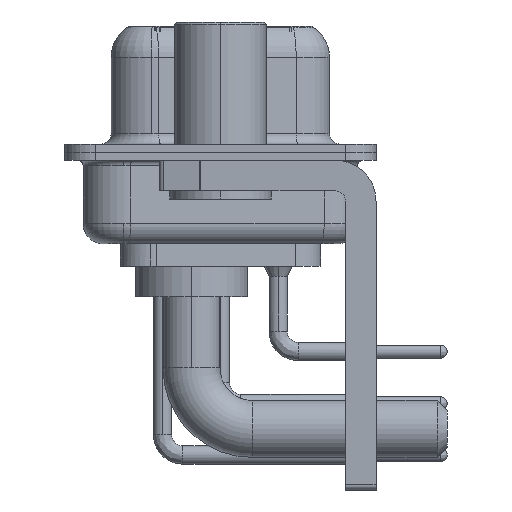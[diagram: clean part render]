
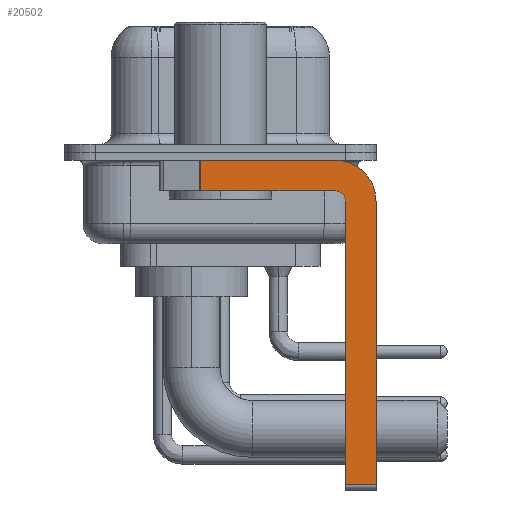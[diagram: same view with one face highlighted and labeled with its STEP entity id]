
A CAD part, left-side view. The second image highlights one B-rep face of the part: STEP entity #20502.
In plain terms, the highlighted planar face has unit normal (-1, 0, 0).
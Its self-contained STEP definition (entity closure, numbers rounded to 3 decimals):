
#913 = DIRECTION ( 'NONE',  ( 0., -1., 0. ) ) ;
#934 = EDGE_CURVE ( 'NONE', #23115, #18921, #5626, .T. ) ;
#1726 = LINE ( 'NONE', #9877, #5058 ) ;
#2110 = VECTOR ( 'NONE', #8054, 1000. ) ;
#2302 = CARTESIAN_POINT ( 'NONE',  ( -2.9, 0.978, -1.9 ) ) ;
#2614 = PLANE ( 'NONE',  #9915 ) ;
#3159 = CARTESIAN_POINT ( 'NONE',  ( -2.9, -7.65, -2.4 ) ) ;
#3480 = CARTESIAN_POINT ( 'NONE',  ( -2.9, -6.15, -16.35 ) ) ;
#3906 = LINE ( 'NONE', #9406, #14219 ) ;
#4399 = DIRECTION ( 'NONE',  ( -1., 0., 0. ) ) ;
#5058 = VECTOR ( 'NONE', #31513, 1000. ) ;
#5063 = ORIENTED_EDGE ( 'NONE', *, *, #16110, .F. ) ;
#5534 = ORIENTED_EDGE ( 'NONE', *, *, #23836, .F. ) ;
#5611 = ORIENTED_EDGE ( 'NONE', *, *, #25659, .F. ) ;
#5626 = LINE ( 'NONE', #13960, #27375 ) ;
#6168 = LINE ( 'NONE', #3159, #31356 ) ;
#7317 = EDGE_CURVE ( 'NONE', #24608, #19240, #34687, .T. ) ;
#7990 = DIRECTION ( 'NONE',  ( 0., 0., -1. ) ) ;
#8054 = DIRECTION ( 'NONE',  ( 0., 0., 1. ) ) ;
#9406 = CARTESIAN_POINT ( 'NONE',  ( -2.9, 3., -0.4 ) ) ;
#9877 = CARTESIAN_POINT ( 'NONE',  ( -2.9, -5.65, -1.9 ) ) ;
#9915 = AXIS2_PLACEMENT_3D ( 'NONE', #18943, #29733, #31865 ) ;
#12101 = ORIENTED_EDGE ( 'NONE', *, *, #7317, .T. ) ;
#12862 = LINE ( 'NONE', #24046, #2110 ) ;
#13932 = ORIENTED_EDGE ( 'NONE', *, *, #934, .T. ) ;
#13960 = CARTESIAN_POINT ( 'NONE',  ( -2.9, 0.978, -1.9 ) ) ;
#14006 = VERTEX_POINT ( 'NONE', #34419 ) ;
#14129 = DIRECTION ( 'NONE',  ( 0., 0., -1. ) ) ;
#14219 = VECTOR ( 'NONE', #913, 1000. ) ;
#14566 = CIRCLE ( 'NONE', #28159, 0.5 ) ;
#15755 = VECTOR ( 'NONE', #21607, 1000. ) ;
#16110 = EDGE_CURVE ( 'NONE', #17334, #19240, #6168, .T. ) ;
#16821 = ORIENTED_EDGE ( 'NONE', *, *, #33903, .F. ) ;
#17334 = VERTEX_POINT ( 'NONE', #33300 ) ;
#18102 = EDGE_CURVE ( 'NONE', #26642, #17334, #23600, .T. ) ;
#18494 = AXIS2_PLACEMENT_3D ( 'NONE', #18732, #32341, #29512 ) ;
#18732 = CARTESIAN_POINT ( 'NONE',  ( -2.9, -5.65, -2.4 ) ) ;
#18921 = VERTEX_POINT ( 'NONE', #2302 ) ;
#18943 = CARTESIAN_POINT ( 'NONE',  ( -2.9, -5.65, -2.4 ) ) ;
#19240 = VERTEX_POINT ( 'NONE', #24392 ) ;
#20289 = EDGE_LOOP ( 'NONE', ( #16821, #13932, #30147, #5611, #5534, #12101, #5063, #31470 ) ) ;
#20502 = ADVANCED_FACE ( 'NONE', ( #21083 ), #2614, .F. ) ;
#20661 = CARTESIAN_POINT ( 'NONE',  ( -2.9, -5.65, -0.4 ) ) ;
#21083 = FACE_OUTER_BOUND ( 'NONE', #20289, .T. ) ;
#21110 = CARTESIAN_POINT ( 'NONE',  ( -2.9, -5.65, -2.4 ) ) ;
#21607 = DIRECTION ( 'NONE',  ( 0., -1., 0. ) ) ;
#23115 = VERTEX_POINT ( 'NONE', #23238 ) ;
#23238 = CARTESIAN_POINT ( 'NONE',  ( -2.9, 0.978, -0.4 ) ) ;
#23600 = CIRCLE ( 'NONE', #18494, 2. ) ;
#23836 = EDGE_CURVE ( 'NONE', #24608, #14006, #12862, .T. ) ;
#24046 = CARTESIAN_POINT ( 'NONE',  ( -2.9, -6.15, -16.6 ) ) ;
#24048 = VERTEX_POINT ( 'NONE', #29818 ) ;
#24392 = CARTESIAN_POINT ( 'NONE',  ( -2.9, -7.65, -16.35 ) ) ;
#24608 = VERTEX_POINT ( 'NONE', #3480 ) ;
#25659 = EDGE_CURVE ( 'NONE', #14006, #24048, #14566, .T. ) ;
#26366 = CARTESIAN_POINT ( 'NONE',  ( -2.9, -5.65, -16.35 ) ) ;
#26642 = VERTEX_POINT ( 'NONE', #20661 ) ;
#27375 = VECTOR ( 'NONE', #14129, 1000. ) ;
#28159 = AXIS2_PLACEMENT_3D ( 'NONE', #21110, #4399, #31890 ) ;
#29066 = EDGE_CURVE ( 'NONE', #24048, #18921, #1726, .T. ) ;
#29512 = DIRECTION ( 'NONE',  ( 0., 0., -1. ) ) ;
#29733 = DIRECTION ( 'NONE',  ( 1., 0., 0. ) ) ;
#29818 = CARTESIAN_POINT ( 'NONE',  ( -2.9, -5.65, -1.9 ) ) ;
#30147 = ORIENTED_EDGE ( 'NONE', *, *, #29066, .F. ) ;
#31356 = VECTOR ( 'NONE', #7990, 1000. ) ;
#31470 = ORIENTED_EDGE ( 'NONE', *, *, #18102, .F. ) ;
#31513 = DIRECTION ( 'NONE',  ( 0., 1., 0. ) ) ;
#31865 = DIRECTION ( 'NONE',  ( 0., 0., -1. ) ) ;
#31890 = DIRECTION ( 'NONE',  ( 0., 0., 1. ) ) ;
#32341 = DIRECTION ( 'NONE',  ( 1., 0., 0. ) ) ;
#33300 = CARTESIAN_POINT ( 'NONE',  ( -2.9, -7.65, -2.4 ) ) ;
#33903 = EDGE_CURVE ( 'NONE', #23115, #26642, #3906, .T. ) ;
#34419 = CARTESIAN_POINT ( 'NONE',  ( -2.9, -6.15, -2.4 ) ) ;
#34687 = LINE ( 'NONE', #26366, #15755 ) ;
